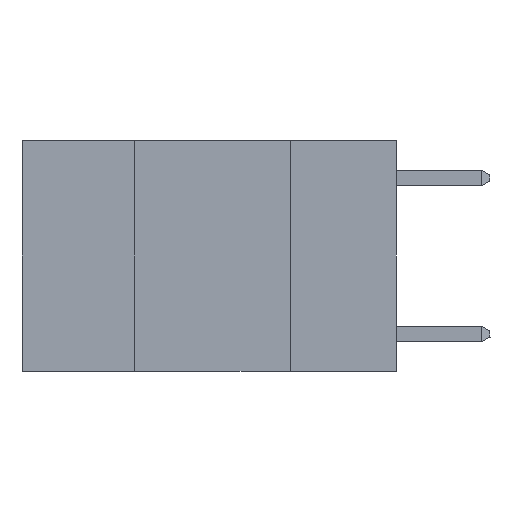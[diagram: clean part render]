
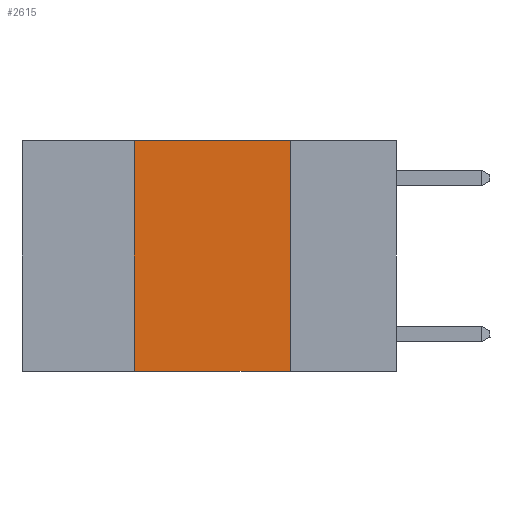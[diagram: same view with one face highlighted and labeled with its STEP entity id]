
A CAD part, left-side view. The second image highlights one B-rep face of the part: STEP entity #2615.
In plain terms, the highlighted planar face has unit normal (-1, 0, 0).
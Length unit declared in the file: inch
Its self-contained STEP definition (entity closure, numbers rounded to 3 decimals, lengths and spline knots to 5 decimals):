
#603 = DIRECTION ( 'NONE',  ( 0., -1., 0. ) ) ;
#957 = LINE ( 'NONE', #4096, #5894 ) ;
#1564 = AXIS2_PLACEMENT_3D ( 'NONE', #8076, #10533, #3401 ) ;
#2615 = ADVANCED_FACE ( 'NONE', ( #18206 ), #12954, .F. ) ;
#3401 = DIRECTION ( 'NONE',  ( 0., 0., -1. ) ) ;
#3548 = VERTEX_POINT ( 'NONE', #11903 ) ;
#4096 = CARTESIAN_POINT ( 'NONE',  ( 0., 0.6, -0.37 ) ) ;
#4187 = VECTOR ( 'NONE', #12924, 39.37008 ) ;
#5894 = VECTOR ( 'NONE', #17852, 39.37008 ) ;
#6035 = CARTESIAN_POINT ( 'NONE',  ( 0., 0.17, 0. ) ) ;
#6619 = VECTOR ( 'NONE', #9936, 39.37008 ) ;
#6976 = CARTESIAN_POINT ( 'NONE',  ( 0., 0.42, 0. ) ) ;
#7750 = VECTOR ( 'NONE', #603, 39.37008 ) ;
#7850 = LINE ( 'NONE', #14741, #7750 ) ;
#8076 = CARTESIAN_POINT ( 'NONE',  ( 0., 0.6, 0. ) ) ;
#8514 = ORIENTED_EDGE ( 'NONE', *, *, #19319, .F. ) ;
#9401 = LINE ( 'NONE', #6976, #4187 ) ;
#9936 = DIRECTION ( 'NONE',  ( 0., 0., -1. ) ) ;
#10533 = DIRECTION ( 'NONE',  ( 1., 0., 0. ) ) ;
#10788 = EDGE_CURVE ( 'NONE', #3548, #14149, #7850, .T. ) ;
#11103 = VERTEX_POINT ( 'NONE', #13783 ) ;
#11903 = CARTESIAN_POINT ( 'NONE',  ( 0., 0.42, 0. ) ) ;
#11981 = CARTESIAN_POINT ( 'NONE',  ( 0., 0.17, 0. ) ) ;
#12924 = DIRECTION ( 'NONE',  ( 0., 0., 1. ) ) ;
#12954 = PLANE ( 'NONE',  #1564 ) ;
#13783 = CARTESIAN_POINT ( 'NONE',  ( 0., 0.42, -0.37 ) ) ;
#14114 = VERTEX_POINT ( 'NONE', #17686 ) ;
#14146 = EDGE_CURVE ( 'NONE', #14149, #14114, #17083, .T. ) ;
#14149 = VERTEX_POINT ( 'NONE', #11981 ) ;
#14741 = CARTESIAN_POINT ( 'NONE',  ( 0., 0.6, 0. ) ) ;
#17083 = LINE ( 'NONE', #6035, #6619 ) ;
#17570 = EDGE_CURVE ( 'NONE', #11103, #14114, #957, .T. ) ;
#17686 = CARTESIAN_POINT ( 'NONE',  ( 0., 0.17, -0.37 ) ) ;
#17852 = DIRECTION ( 'NONE',  ( 0., -1., 0. ) ) ;
#18206 = FACE_OUTER_BOUND ( 'NONE', #23535, .T. ) ;
#19016 = ORIENTED_EDGE ( 'NONE', *, *, #14146, .F. ) ;
#19319 = EDGE_CURVE ( 'NONE', #11103, #3548, #9401, .T. ) ;
#21327 = ORIENTED_EDGE ( 'NONE', *, *, #10788, .F. ) ;
#22992 = ORIENTED_EDGE ( 'NONE', *, *, #17570, .T. ) ;
#23535 = EDGE_LOOP ( 'NONE', ( #19016, #21327, #8514, #22992 ) ) ;
